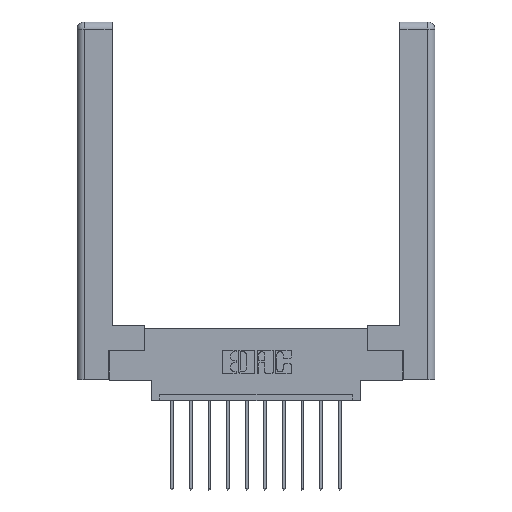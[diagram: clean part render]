
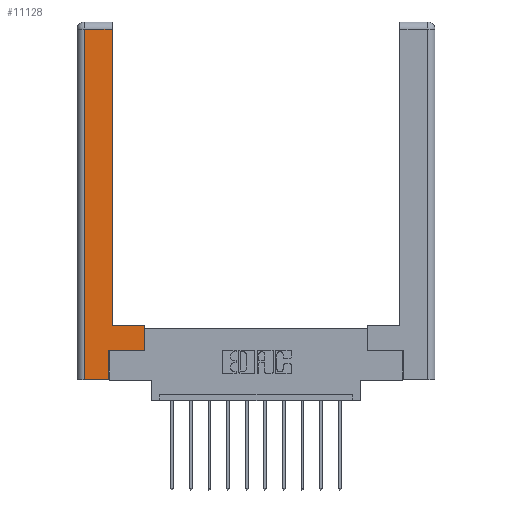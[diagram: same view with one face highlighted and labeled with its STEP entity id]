
A CAD part, top view. The second image highlights one B-rep face of the part: STEP entity #11128.
In plain terms, the highlighted planar face has unit normal (0, 0, 1).
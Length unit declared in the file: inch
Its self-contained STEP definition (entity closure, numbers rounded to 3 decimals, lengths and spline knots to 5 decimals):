
#524 = ORIENTED_EDGE ( 'NONE', *, *, #5786, .T. ) ;
#636 = VERTEX_POINT ( 'NONE', #3256 ) ;
#717 = VECTOR ( 'NONE', #6151, 39.37008 ) ;
#1035 = VECTOR ( 'NONE', #13896, 39.37008 ) ;
#1160 = VECTOR ( 'NONE', #9801, 39.37008 ) ;
#1185 = VERTEX_POINT ( 'NONE', #5174 ) ;
#1291 = DIRECTION ( 'NONE',  ( 0., 1., 0. ) ) ;
#1709 = CARTESIAN_POINT ( 'NONE',  ( 0.295, 2.94, 0. ) ) ;
#2078 = LINE ( 'NONE', #13196, #8469 ) ;
#2251 = VECTOR ( 'NONE', #3599, 39.37008 ) ;
#2332 = VERTEX_POINT ( 'NONE', #1709 ) ;
#2744 = ORIENTED_EDGE ( 'NONE', *, *, #6509, .T. ) ;
#3249 = DIRECTION ( 'NONE',  ( -1., 0., 0. ) ) ;
#3256 = CARTESIAN_POINT ( 'NONE',  ( 0.0615, 0., 0. ) ) ;
#3285 = EDGE_CURVE ( 'NONE', #1185, #636, #7981, .T. ) ;
#3516 = FACE_OUTER_BOUND ( 'NONE', #12142, .T. ) ;
#3599 = DIRECTION ( 'NONE',  ( -1., 0., 0. ) ) ;
#3624 = LINE ( 'NONE', #8224, #1035 ) ;
#3814 = VECTOR ( 'NONE', #6975, 39.37008 ) ;
#5174 = CARTESIAN_POINT ( 'NONE',  ( 0.0615, 2.94, 0. ) ) ;
#5191 = CARTESIAN_POINT ( 'NONE',  ( 0.0615, 2.94, 0. ) ) ;
#5786 = EDGE_CURVE ( 'NONE', #2332, #1185, #13368, .T. ) ;
#5839 = CARTESIAN_POINT ( 'NONE',  ( 0.295, 3., 0. ) ) ;
#6151 = DIRECTION ( 'NONE',  ( -1., 0., 0. ) ) ;
#6509 = EDGE_CURVE ( 'NONE', #12192, #11883, #3624, .T. ) ;
#6589 = LINE ( 'NONE', #11218, #2251 ) ;
#6975 = DIRECTION ( 'NONE',  ( 1., 0., 0. ) ) ;
#7752 = CARTESIAN_POINT ( 'NONE',  ( 0.265, 0., 0. ) ) ;
#7817 = VERTEX_POINT ( 'NONE', #11888 ) ;
#7862 = ORIENTED_EDGE ( 'NONE', *, *, #9004, .T. ) ;
#7981 = LINE ( 'NONE', #9492, #9014 ) ;
#8082 = CARTESIAN_POINT ( 'NONE',  ( 0.565, 0.245, 0. ) ) ;
#8224 = CARTESIAN_POINT ( 'NONE',  ( 0.265, 0.245, 0. ) ) ;
#8238 = LINE ( 'NONE', #9836, #1160 ) ;
#8240 = VERTEX_POINT ( 'NONE', #12932 ) ;
#8446 = CARTESIAN_POINT ( 'NONE',  ( 0.265, 0.245, 0. ) ) ;
#8469 = VECTOR ( 'NONE', #1291, 39.37008 ) ;
#8765 = CARTESIAN_POINT ( 'NONE',  ( 0., 0., 0. ) ) ;
#8837 = ORIENTED_EDGE ( 'NONE', *, *, #9351, .T. ) ;
#8847 = DIRECTION ( 'NONE',  ( 0., 0., -1. ) ) ;
#8943 = PLANE ( 'NONE',  #14324 ) ;
#8971 = EDGE_CURVE ( 'NONE', #11883, #13781, #11927, .T. ) ;
#9004 = EDGE_CURVE ( 'NONE', #8240, #7817, #6589, .T. ) ;
#9014 = VECTOR ( 'NONE', #12912, 39.37008 ) ;
#9054 = DIRECTION ( 'NONE',  ( 0., 1., 0. ) ) ;
#9351 = EDGE_CURVE ( 'NONE', #13781, #8240, #2078, .T. ) ;
#9461 = EDGE_CURVE ( 'NONE', #7817, #2332, #14375, .T. ) ;
#9492 = CARTESIAN_POINT ( 'NONE',  ( 0.0615, 0., 0. ) ) ;
#9631 = ORIENTED_EDGE ( 'NONE', *, *, #8971, .T. ) ;
#9801 = DIRECTION ( 'NONE',  ( 1., 0., 0. ) ) ;
#9836 = CARTESIAN_POINT ( 'NONE',  ( 0.265, 0., 0. ) ) ;
#10005 = ORIENTED_EDGE ( 'NONE', *, *, #3285, .T. ) ;
#10419 = ORIENTED_EDGE ( 'NONE', *, *, #9461, .T. ) ;
#11128 = ADVANCED_FACE ( 'NONE', ( #3516 ), #8943, .F. ) ;
#11218 = CARTESIAN_POINT ( 'NONE',  ( 0.295, 0.45, 0. ) ) ;
#11883 = VERTEX_POINT ( 'NONE', #8446 ) ;
#11888 = CARTESIAN_POINT ( 'NONE',  ( 0.295, 0.45, 0. ) ) ;
#11927 = LINE ( 'NONE', #8082, #3814 ) ;
#12056 = ORIENTED_EDGE ( 'NONE', *, *, #14248, .T. ) ;
#12142 = EDGE_LOOP ( 'NONE', ( #10419, #524, #10005, #12056, #2744, #9631, #8837, #7862 ) ) ;
#12192 = VERTEX_POINT ( 'NONE', #7752 ) ;
#12441 = VECTOR ( 'NONE', #9054, 39.37008 ) ;
#12912 = DIRECTION ( 'NONE',  ( 0., -1., 0. ) ) ;
#12932 = CARTESIAN_POINT ( 'NONE',  ( 0.565, 0.45, 0. ) ) ;
#13196 = CARTESIAN_POINT ( 'NONE',  ( 0.565, 0.45, 0. ) ) ;
#13368 = LINE ( 'NONE', #5191, #717 ) ;
#13460 = CARTESIAN_POINT ( 'NONE',  ( 0.565, 0.245, 0. ) ) ;
#13781 = VERTEX_POINT ( 'NONE', #13460 ) ;
#13896 = DIRECTION ( 'NONE',  ( 0., 1., 0. ) ) ;
#14248 = EDGE_CURVE ( 'NONE', #636, #12192, #8238, .T. ) ;
#14324 = AXIS2_PLACEMENT_3D ( 'NONE', #8765, #8847, #3249 ) ;
#14375 = LINE ( 'NONE', #5839, #12441 ) ;
